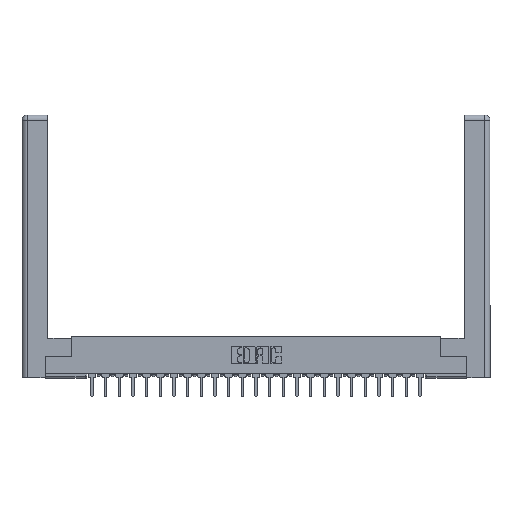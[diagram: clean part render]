
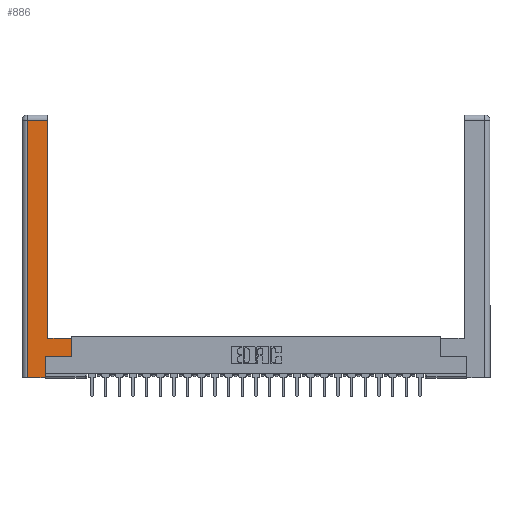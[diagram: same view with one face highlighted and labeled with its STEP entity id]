
A CAD part, top view. The second image highlights one B-rep face of the part: STEP entity #886.
In plain terms, the highlighted planar face has unit normal (0, 0, 1).
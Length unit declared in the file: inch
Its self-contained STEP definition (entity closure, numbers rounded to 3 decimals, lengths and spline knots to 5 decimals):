
#753 = AXIS2_PLACEMENT_3D ( 'NONE', #18904, #6105, #8138 ) ;
#886 = ADVANCED_FACE ( 'NONE', ( #24207 ), #14833, .F. ) ;
#1585 = ORIENTED_EDGE ( 'NONE', *, *, #21225, .T. ) ;
#1645 = VECTOR ( 'NONE', #25775, 39.37008 ) ;
#1963 = DIRECTION ( 'NONE',  ( 0., 1., 0. ) ) ;
#2365 = DIRECTION ( 'NONE',  ( 0., 1., 0. ) ) ;
#2719 = VECTOR ( 'NONE', #15124, 39.37008 ) ;
#3856 = CARTESIAN_POINT ( 'NONE',  ( 0.0615, 2.94, 0. ) ) ;
#4089 = LINE ( 'NONE', #23148, #21740 ) ;
#4170 = VECTOR ( 'NONE', #2365, 39.37008 ) ;
#4631 = LINE ( 'NONE', #8324, #24475 ) ;
#5500 = CARTESIAN_POINT ( 'NONE',  ( 0.0615, 0., 0. ) ) ;
#6105 = DIRECTION ( 'NONE',  ( 0., 0., -1. ) ) ;
#6372 = VECTOR ( 'NONE', #1963, 39.37008 ) ;
#6401 = CARTESIAN_POINT ( 'NONE',  ( 0.0615, 2.94, 0. ) ) ;
#6592 = EDGE_CURVE ( 'NONE', #14817, #24616, #4089, .T. ) ;
#6599 = VERTEX_POINT ( 'NONE', #19183 ) ;
#7282 = DIRECTION ( 'NONE',  ( 1., 0., 0. ) ) ;
#8138 = DIRECTION ( 'NONE',  ( -1., 0., 0. ) ) ;
#8324 = CARTESIAN_POINT ( 'NONE',  ( 0.265, 0., 0. ) ) ;
#9760 = LINE ( 'NONE', #12532, #18572 ) ;
#10195 = CARTESIAN_POINT ( 'NONE',  ( 0.295, 3., 0. ) ) ;
#10207 = LINE ( 'NONE', #3856, #14278 ) ;
#11752 = EDGE_LOOP ( 'NONE', ( #13036, #13191, #14778, #21855, #25091, #12732, #1585, #22315 ) ) ;
#12497 = VERTEX_POINT ( 'NONE', #23387 ) ;
#12530 = EDGE_CURVE ( 'NONE', #18431, #12497, #25255, .T. ) ;
#12532 = CARTESIAN_POINT ( 'NONE',  ( 0.265, 0.245, 0. ) ) ;
#12732 = ORIENTED_EDGE ( 'NONE', *, *, #6592, .T. ) ;
#12756 = CARTESIAN_POINT ( 'NONE',  ( 0.295, 0.45, 0. ) ) ;
#12886 = VERTEX_POINT ( 'NONE', #22382 ) ;
#13036 = ORIENTED_EDGE ( 'NONE', *, *, #21954, .T. ) ;
#13191 = ORIENTED_EDGE ( 'NONE', *, *, #20501, .T. ) ;
#14278 = VECTOR ( 'NONE', #19867, 39.37008 ) ;
#14753 = EDGE_CURVE ( 'NONE', #12497, #21352, #4631, .T. ) ;
#14778 = ORIENTED_EDGE ( 'NONE', *, *, #12530, .T. ) ;
#14817 = VERTEX_POINT ( 'NONE', #24615 ) ;
#14833 = PLANE ( 'NONE',  #753 ) ;
#15124 = DIRECTION ( 'NONE',  ( -1., 0., 0. ) ) ;
#16465 = DIRECTION ( 'NONE',  ( 0., 1., 0. ) ) ;
#17103 = LINE ( 'NONE', #18061, #6372 ) ;
#18061 = CARTESIAN_POINT ( 'NONE',  ( 0.565, 0.45, 0. ) ) ;
#18431 = VERTEX_POINT ( 'NONE', #6401 ) ;
#18572 = VECTOR ( 'NONE', #16465, 39.37008 ) ;
#18816 = DIRECTION ( 'NONE',  ( 1., 0., 0. ) ) ;
#18904 = CARTESIAN_POINT ( 'NONE',  ( 0., 0., 0. ) ) ;
#19183 = CARTESIAN_POINT ( 'NONE',  ( 0.295, 2.94, 0. ) ) ;
#19397 = CARTESIAN_POINT ( 'NONE',  ( 0.565, 0.45, 0. ) ) ;
#19531 = EDGE_CURVE ( 'NONE', #20972, #12886, #23515, .T. ) ;
#19867 = DIRECTION ( 'NONE',  ( -1., 0., 0. ) ) ;
#20501 = EDGE_CURVE ( 'NONE', #6599, #18431, #10207, .T. ) ;
#20972 = VERTEX_POINT ( 'NONE', #19397 ) ;
#21225 = EDGE_CURVE ( 'NONE', #24616, #20972, #17103, .T. ) ;
#21352 = VERTEX_POINT ( 'NONE', #24643 ) ;
#21740 = VECTOR ( 'NONE', #7282, 39.37008 ) ;
#21855 = ORIENTED_EDGE ( 'NONE', *, *, #14753, .T. ) ;
#21954 = EDGE_CURVE ( 'NONE', #12886, #6599, #25261, .T. ) ;
#22315 = ORIENTED_EDGE ( 'NONE', *, *, #19531, .T. ) ;
#22382 = CARTESIAN_POINT ( 'NONE',  ( 0.295, 0.45, 0. ) ) ;
#22737 = EDGE_CURVE ( 'NONE', #21352, #14817, #9760, .T. ) ;
#23148 = CARTESIAN_POINT ( 'NONE',  ( 0.565, 0.245, 0. ) ) ;
#23387 = CARTESIAN_POINT ( 'NONE',  ( 0.0615, 0., 0. ) ) ;
#23515 = LINE ( 'NONE', #12756, #2719 ) ;
#24207 = FACE_OUTER_BOUND ( 'NONE', #11752, .T. ) ;
#24475 = VECTOR ( 'NONE', #18816, 39.37008 ) ;
#24615 = CARTESIAN_POINT ( 'NONE',  ( 0.265, 0.245, 0. ) ) ;
#24616 = VERTEX_POINT ( 'NONE', #24934 ) ;
#24643 = CARTESIAN_POINT ( 'NONE',  ( 0.265, 0., 0. ) ) ;
#24934 = CARTESIAN_POINT ( 'NONE',  ( 0.565, 0.245, 0. ) ) ;
#25091 = ORIENTED_EDGE ( 'NONE', *, *, #22737, .T. ) ;
#25255 = LINE ( 'NONE', #5500, #1645 ) ;
#25261 = LINE ( 'NONE', #10195, #4170 ) ;
#25775 = DIRECTION ( 'NONE',  ( 0., -1., 0. ) ) ;
